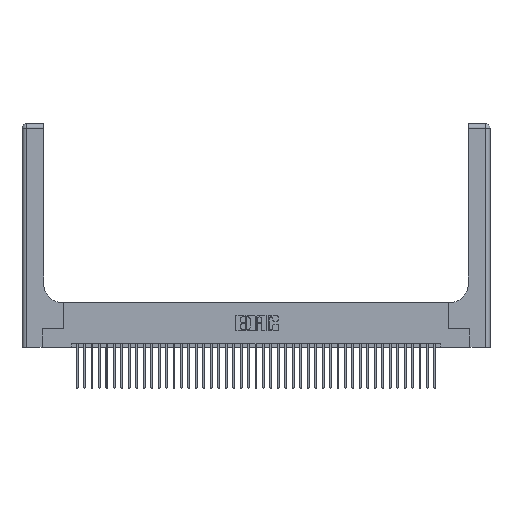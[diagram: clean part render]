
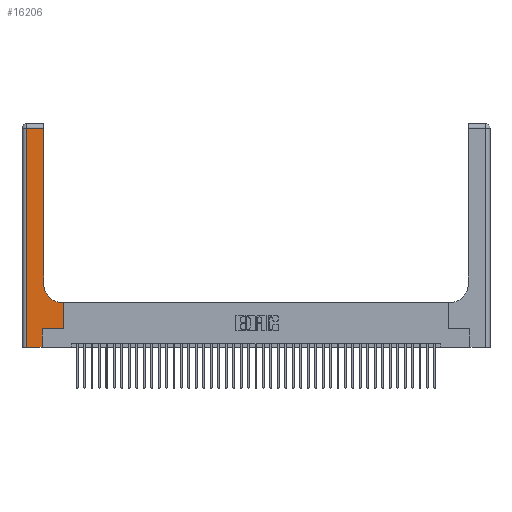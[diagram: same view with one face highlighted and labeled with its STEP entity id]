
A CAD part, top view. The second image highlights one B-rep face of the part: STEP entity #16206.
In plain terms, the highlighted planar face has unit normal (0, 0, 1).
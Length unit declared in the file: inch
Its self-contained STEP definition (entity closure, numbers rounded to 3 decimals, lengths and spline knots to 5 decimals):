
#2535 = CARTESIAN_POINT ( 'NONE',  ( 0.269, 0.25, 0.37 ) ) ;
#2685 = VERTEX_POINT ( 'NONE', #25293 ) ;
#2693 = ORIENTED_EDGE ( 'NONE', *, *, #12502, .T. ) ;
#3180 = EDGE_CURVE ( 'NONE', #25674, #22031, #24391, .T. ) ;
#4859 = LINE ( 'NONE', #14197, #42534 ) ;
#5239 = ORIENTED_EDGE ( 'NONE', *, *, #10091, .T. ) ;
#5656 = LINE ( 'NONE', #2535, #17983 ) ;
#6077 = CARTESIAN_POINT ( 'NONE',  ( 0.5415, 0.85, 0.37 ) ) ;
#6427 = ORIENTED_EDGE ( 'NONE', *, *, #8320, .T. ) ;
#6497 = PLANE ( 'NONE',  #9856 ) ;
#6505 = DIRECTION ( 'NONE',  ( 1., 0., 0. ) ) ;
#7011 = DIRECTION ( 'NONE',  ( 0., 1., 0. ) ) ;
#7098 = DIRECTION ( 'NONE',  ( 0., 1., 0. ) ) ;
#7244 = CARTESIAN_POINT ( 'NONE',  ( 0.5585, 0.25, 0.37 ) ) ;
#8320 = EDGE_CURVE ( 'NONE', #16274, #11762, #27746, .T. ) ;
#8403 = DIRECTION ( 'NONE',  ( -1., 0., 0. ) ) ;
#8773 = VERTEX_POINT ( 'NONE', #30196 ) ;
#8908 = ORIENTED_EDGE ( 'NONE', *, *, #13547, .T. ) ;
#9856 = AXIS2_PLACEMENT_3D ( 'NONE', #12823, #39356, #29562 ) ;
#10091 = EDGE_CURVE ( 'NONE', #2685, #37040, #41103, .T. ) ;
#11576 = CARTESIAN_POINT ( 'NONE',  ( 0.5415, 0.6, 0.37 ) ) ;
#11762 = VERTEX_POINT ( 'NONE', #11576 ) ;
#11913 = VECTOR ( 'NONE', #7098, 39.37008 ) ;
#12186 = VECTOR ( 'NONE', #25133, 39.37008 ) ;
#12370 = CIRCLE ( 'NONE', #32883, 0.25 ) ;
#12502 = EDGE_CURVE ( 'NONE', #35143, #8773, #31797, .T. ) ;
#12823 = CARTESIAN_POINT ( 'NONE',  ( 0., 3., 0.37 ) ) ;
#13477 = CARTESIAN_POINT ( 'NONE',  ( 0.2915, 3., 0.37 ) ) ;
#13547 = EDGE_CURVE ( 'NONE', #22031, #2685, #4859, .T. ) ;
#13742 = CARTESIAN_POINT ( 'NONE',  ( 0.5585, 0.6, 0.37 ) ) ;
#14197 = CARTESIAN_POINT ( 'NONE',  ( 0., 0., 0.37 ) ) ;
#14306 = ORIENTED_EDGE ( 'NONE', *, *, #39573, .T. ) ;
#16206 = ADVANCED_FACE ( 'NONE', ( #31048 ), #6497, .F. ) ;
#16274 = VERTEX_POINT ( 'NONE', #13742 ) ;
#17003 = CARTESIAN_POINT ( 'NONE',  ( 0.06, 3., 0.37 ) ) ;
#17528 = ORIENTED_EDGE ( 'NONE', *, *, #27828, .T. ) ;
#17983 = VECTOR ( 'NONE', #28780, 39.37008 ) ;
#18049 = ORIENTED_EDGE ( 'NONE', *, *, #41812, .T. ) ;
#18051 = CARTESIAN_POINT ( 'NONE',  ( 0.2915, 0.85, 0.37 ) ) ;
#19464 = DIRECTION ( 'NONE',  ( 0., 0., -1. ) ) ;
#19854 = ORIENTED_EDGE ( 'NONE', *, *, #3180, .T. ) ;
#21586 = ORIENTED_EDGE ( 'NONE', *, *, #33264, .T. ) ;
#22031 = VERTEX_POINT ( 'NONE', #31256 ) ;
#23566 = CARTESIAN_POINT ( 'NONE',  ( 0.269, 0., 0.37 ) ) ;
#24391 = LINE ( 'NONE', #17003, #31121 ) ;
#24827 = CARTESIAN_POINT ( 'NONE',  ( 0.269, 0.25, 0.37 ) ) ;
#24981 = CARTESIAN_POINT ( 'NONE',  ( 0., 2.94, 0.37 ) ) ;
#25090 = VERTEX_POINT ( 'NONE', #30409 ) ;
#25133 = DIRECTION ( 'NONE',  ( 0., 1., 0. ) ) ;
#25293 = CARTESIAN_POINT ( 'NONE',  ( 0.269, 0., 0.37 ) ) ;
#25674 = VERTEX_POINT ( 'NONE', #32935 ) ;
#27746 = LINE ( 'NONE', #33831, #32940 ) ;
#27828 = EDGE_CURVE ( 'NONE', #25090, #16274, #37173, .T. ) ;
#28780 = DIRECTION ( 'NONE',  ( 1., 0., 0. ) ) ;
#29562 = DIRECTION ( 'NONE',  ( -1., 0., 0. ) ) ;
#30196 = CARTESIAN_POINT ( 'NONE',  ( 0.2915, 2.94, 0.37 ) ) ;
#30409 = CARTESIAN_POINT ( 'NONE',  ( 0.5585, 0.25, 0.37 ) ) ;
#30783 = VECTOR ( 'NONE', #7011, 39.37008 ) ;
#31048 = FACE_OUTER_BOUND ( 'NONE', #40323, .T. ) ;
#31121 = VECTOR ( 'NONE', #36918, 39.37008 ) ;
#31256 = CARTESIAN_POINT ( 'NONE',  ( 0.06, 0., 0.37 ) ) ;
#31797 = LINE ( 'NONE', #13477, #12186 ) ;
#31804 = DIRECTION ( 'NONE',  ( 1., 0., 0. ) ) ;
#32316 = VECTOR ( 'NONE', #8403, 39.37008 ) ;
#32883 = AXIS2_PLACEMENT_3D ( 'NONE', #6077, #19464, #6505 ) ;
#32935 = CARTESIAN_POINT ( 'NONE',  ( 0.06, 2.94, 0.37 ) ) ;
#32940 = VECTOR ( 'NONE', #40469, 39.37008 ) ;
#33264 = EDGE_CURVE ( 'NONE', #37040, #25090, #5656, .T. ) ;
#33831 = CARTESIAN_POINT ( 'NONE',  ( 0.2915, 0.6, 0.37 ) ) ;
#35143 = VERTEX_POINT ( 'NONE', #18051 ) ;
#36918 = DIRECTION ( 'NONE',  ( 0., -1., 0. ) ) ;
#37040 = VERTEX_POINT ( 'NONE', #24827 ) ;
#37173 = LINE ( 'NONE', #7244, #11913 ) ;
#38528 = LINE ( 'NONE', #24981, #32316 ) ;
#39356 = DIRECTION ( 'NONE',  ( 0., 0., -1. ) ) ;
#39573 = EDGE_CURVE ( 'NONE', #11762, #35143, #12370, .T. ) ;
#40323 = EDGE_LOOP ( 'NONE', ( #2693, #18049, #19854, #8908, #5239, #21586, #17528, #6427, #14306 ) ) ;
#40469 = DIRECTION ( 'NONE',  ( -1., 0., 0. ) ) ;
#41103 = LINE ( 'NONE', #23566, #30783 ) ;
#41812 = EDGE_CURVE ( 'NONE', #8773, #25674, #38528, .T. ) ;
#42534 = VECTOR ( 'NONE', #31804, 39.37008 ) ;
